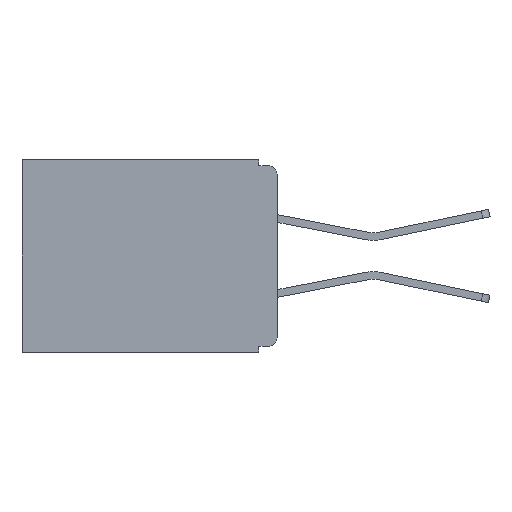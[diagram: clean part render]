
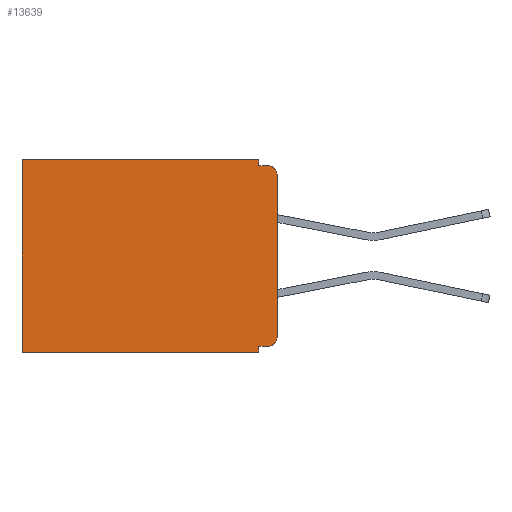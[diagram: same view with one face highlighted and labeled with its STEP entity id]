
A CAD part, left-side view. The second image highlights one B-rep face of the part: STEP entity #13639.
In plain terms, the highlighted planar face has unit normal (-1, 0, 0).
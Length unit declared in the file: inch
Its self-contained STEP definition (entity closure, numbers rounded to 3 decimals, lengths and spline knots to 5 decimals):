
#1357 = ORIENTED_EDGE ( 'NONE', *, *, #17962, .T. ) ;
#1595 = VECTOR ( 'NONE', #18583, 39.37008 ) ;
#2524 = VERTEX_POINT ( 'NONE', #3533 ) ;
#2780 = CARTESIAN_POINT ( 'NONE',  ( 0.3, 0.015, -0.305 ) ) ;
#3533 = CARTESIAN_POINT ( 'NONE',  ( 0.3, 0., -0.305 ) ) ;
#3573 = DIRECTION ( 'NONE',  ( 0., 1., 0. ) ) ;
#3639 = CARTESIAN_POINT ( 'NONE',  ( 0.3, 0.015, -0.025 ) ) ;
#4572 = EDGE_CURVE ( 'NONE', #20848, #21001, #15103, .T. ) ;
#5487 = EDGE_CURVE ( 'NONE', #9615, #18887, #9561, .T. ) ;
#5614 = DIRECTION ( 'NONE',  ( 0., 0., -1. ) ) ;
#6464 = DIRECTION ( 'NONE',  ( 0., 0., -1. ) ) ;
#6608 = VECTOR ( 'NONE', #9273, 39.37008 ) ;
#6990 = PLANE ( 'NONE',  #15638 ) ;
#7120 = DIRECTION ( 'NONE',  ( 1., 0., 0. ) ) ;
#8106 = ORIENTED_EDGE ( 'NONE', *, *, #25013, .T. ) ;
#8585 = ORIENTED_EDGE ( 'NONE', *, *, #4572, .F. ) ;
#8875 = VERTEX_POINT ( 'NONE', #16816 ) ;
#8949 = ORIENTED_EDGE ( 'NONE', *, *, #25851, .F. ) ;
#9273 = DIRECTION ( 'NONE',  ( 0., 0., -1. ) ) ;
#9561 = LINE ( 'NONE', #21017, #16707 ) ;
#9615 = VERTEX_POINT ( 'NONE', #11991 ) ;
#10234 = LINE ( 'NONE', #10503, #16546 ) ;
#10497 = CARTESIAN_POINT ( 'NONE',  ( 0.3, 0.031, 0. ) ) ;
#10503 = CARTESIAN_POINT ( 'NONE',  ( 0.3, 0.437, -0.33 ) ) ;
#10524 = FACE_OUTER_BOUND ( 'NONE', #29741, .T. ) ;
#11631 = CARTESIAN_POINT ( 'NONE',  ( 0.3, 0., -0.32 ) ) ;
#11686 = LINE ( 'NONE', #26345, #32544 ) ;
#11841 = DIRECTION ( 'NONE',  ( 0., -1., 0. ) ) ;
#11991 = CARTESIAN_POINT ( 'NONE',  ( 0.3, 0.031, -0.33 ) ) ;
#12412 = CARTESIAN_POINT ( 'NONE',  ( 0.3, 0.031, -0.32 ) ) ;
#12548 = CARTESIAN_POINT ( 'NONE',  ( 0.3, 0.031, 0. ) ) ;
#13191 = DIRECTION ( 'NONE',  ( 0., 0., -1. ) ) ;
#13221 = DIRECTION ( 'NONE',  ( 0., 0., -1. ) ) ;
#13639 = ADVANCED_FACE ( 'NONE', ( #10524 ), #6990, .F. ) ;
#13824 = LINE ( 'NONE', #27769, #6608 ) ;
#14163 = ORIENTED_EDGE ( 'NONE', *, *, #26755, .F. ) ;
#14323 = DIRECTION ( 'NONE',  ( 0., 1., 0. ) ) ;
#15103 = LINE ( 'NONE', #23865, #29047 ) ;
#15638 = AXIS2_PLACEMENT_3D ( 'NONE', #33370, #7120, #25765 ) ;
#16165 = LINE ( 'NONE', #10497, #1595 ) ;
#16224 = CIRCLE ( 'NONE', #24504, 0.015 ) ;
#16297 = EDGE_CURVE ( 'NONE', #23308, #19793, #21032, .T. ) ;
#16546 = VECTOR ( 'NONE', #13221, 39.37008 ) ;
#16707 = VECTOR ( 'NONE', #29126, 39.37008 ) ;
#16816 = CARTESIAN_POINT ( 'NONE',  ( 0.3, 0., -0.025 ) ) ;
#17168 = CARTESIAN_POINT ( 'NONE',  ( 0.3, 0., 0. ) ) ;
#17962 = EDGE_CURVE ( 'NONE', #24737, #2524, #30977, .T. ) ;
#18352 = ORIENTED_EDGE ( 'NONE', *, *, #16297, .T. ) ;
#18583 = DIRECTION ( 'NONE',  ( 0., 0., -1. ) ) ;
#18887 = VERTEX_POINT ( 'NONE', #27883 ) ;
#19684 = ORIENTED_EDGE ( 'NONE', *, *, #5487, .F. ) ;
#19793 = VERTEX_POINT ( 'NONE', #21211 ) ;
#20848 = VERTEX_POINT ( 'NONE', #33102 ) ;
#21001 = VERTEX_POINT ( 'NONE', #33658 ) ;
#21017 = CARTESIAN_POINT ( 'NONE',  ( 0.3, 0., -0.33 ) ) ;
#21032 = LINE ( 'NONE', #17168, #33959 ) ;
#21211 = CARTESIAN_POINT ( 'NONE',  ( 0.3, 0.437, 0. ) ) ;
#21698 = DIRECTION ( 'NONE',  ( -1., 0., 0. ) ) ;
#22288 = VECTOR ( 'NONE', #14323, 39.37008 ) ;
#22526 = DIRECTION ( 'NONE',  ( -1., 0., 0. ) ) ;
#22603 = EDGE_CURVE ( 'NONE', #8875, #2524, #13824, .T. ) ;
#23305 = ORIENTED_EDGE ( 'NONE', *, *, #22603, .F. ) ;
#23308 = VERTEX_POINT ( 'NONE', #12548 ) ;
#23865 = CARTESIAN_POINT ( 'NONE',  ( 0.3, 0., -0.01 ) ) ;
#24093 = EDGE_CURVE ( 'NONE', #31130, #9615, #11686, .T. ) ;
#24504 = AXIS2_PLACEMENT_3D ( 'NONE', #3639, #22526, #6464 ) ;
#24737 = VERTEX_POINT ( 'NONE', #29002 ) ;
#25013 = EDGE_CURVE ( 'NONE', #8875, #21001, #16224, .T. ) ;
#25765 = DIRECTION ( 'NONE',  ( 0., 0., -1. ) ) ;
#25851 = EDGE_CURVE ( 'NONE', #23308, #20848, #16165, .T. ) ;
#26276 = ORIENTED_EDGE ( 'NONE', *, *, #27577, .T. ) ;
#26345 = CARTESIAN_POINT ( 'NONE',  ( 0.3, 0.031, -0.33 ) ) ;
#26755 = EDGE_CURVE ( 'NONE', #24737, #31130, #29194, .T. ) ;
#27577 = EDGE_CURVE ( 'NONE', #19793, #18887, #10234, .T. ) ;
#27769 = CARTESIAN_POINT ( 'NONE',  ( 0.3, 0., -0.33 ) ) ;
#27883 = CARTESIAN_POINT ( 'NONE',  ( 0.3, 0.437, -0.33 ) ) ;
#28600 = ORIENTED_EDGE ( 'NONE', *, *, #24093, .F. ) ;
#29002 = CARTESIAN_POINT ( 'NONE',  ( 0.3, 0.015, -0.32 ) ) ;
#29047 = VECTOR ( 'NONE', #11841, 39.37008 ) ;
#29126 = DIRECTION ( 'NONE',  ( 0., 1., 0. ) ) ;
#29194 = LINE ( 'NONE', #11631, #22288 ) ;
#29741 = EDGE_LOOP ( 'NONE', ( #23305, #8106, #8585, #8949, #18352, #26276, #19684, #28600, #14163, #1357 ) ) ;
#30977 = CIRCLE ( 'NONE', #32721, 0.015 ) ;
#31130 = VERTEX_POINT ( 'NONE', #12412 ) ;
#32544 = VECTOR ( 'NONE', #13191, 39.37008 ) ;
#32721 = AXIS2_PLACEMENT_3D ( 'NONE', #2780, #21698, #5614 ) ;
#33102 = CARTESIAN_POINT ( 'NONE',  ( 0.3, 0.031, -0.01 ) ) ;
#33370 = CARTESIAN_POINT ( 'NONE',  ( 0.3, 0., -0.33 ) ) ;
#33658 = CARTESIAN_POINT ( 'NONE',  ( 0.3, 0.015, -0.01 ) ) ;
#33959 = VECTOR ( 'NONE', #3573, 39.37008 ) ;
